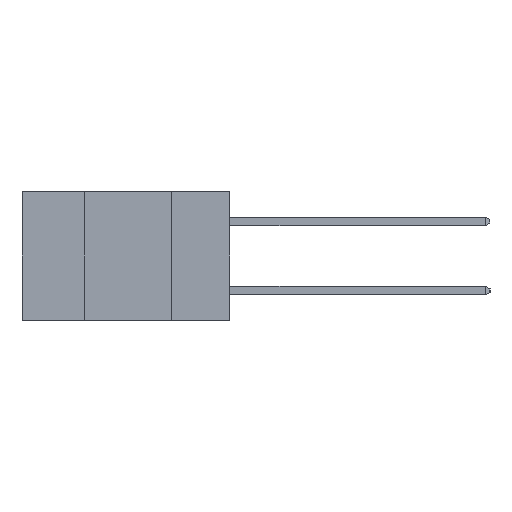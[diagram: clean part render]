
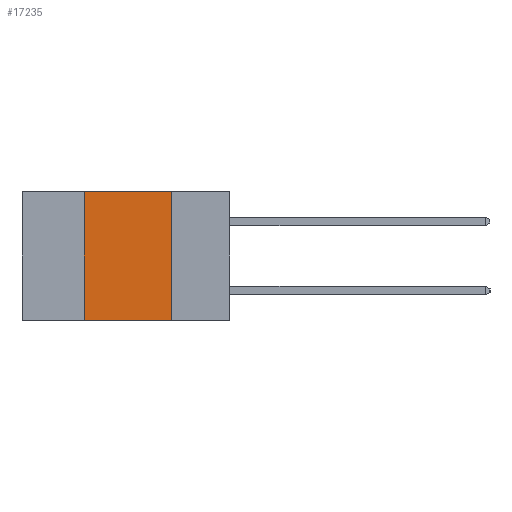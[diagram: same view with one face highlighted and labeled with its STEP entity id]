
A CAD part, left-side view. The second image highlights one B-rep face of the part: STEP entity #17235.
In plain terms, the highlighted planar face has unit normal (-1, 0, 0).
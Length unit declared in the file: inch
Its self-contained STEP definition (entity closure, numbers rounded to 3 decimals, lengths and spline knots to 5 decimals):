
#1787 = CARTESIAN_POINT ( 'NONE',  ( 0., 0.17, -0.37 ) ) ;
#2002 = LINE ( 'NONE', #13239, #11892 ) ;
#2721 = EDGE_CURVE ( 'NONE', #7994, #11828, #11859, .T. ) ;
#3943 = PLANE ( 'NONE',  #11125 ) ;
#5188 = VECTOR ( 'NONE', #9706, 39.37008 ) ;
#5270 = CARTESIAN_POINT ( 'NONE',  ( 0., 0.6, 0. ) ) ;
#5330 = DIRECTION ( 'NONE',  ( 0., 0., -1. ) ) ;
#7045 = ORIENTED_EDGE ( 'NONE', *, *, #13867, .F. ) ;
#7994 = VERTEX_POINT ( 'NONE', #9595 ) ;
#8025 = EDGE_CURVE ( 'NONE', #12094, #7994, #15851, .T. ) ;
#8326 = VECTOR ( 'NONE', #8555, 39.37008 ) ;
#8513 = CARTESIAN_POINT ( 'NONE',  ( 0., 0.6, 0. ) ) ;
#8555 = DIRECTION ( 'NONE',  ( 0., -1., 0. ) ) ;
#9113 = VERTEX_POINT ( 'NONE', #10528 ) ;
#9206 = LINE ( 'NONE', #1787, #12334 ) ;
#9595 = CARTESIAN_POINT ( 'NONE',  ( 0., 0.42, 0. ) ) ;
#9706 = DIRECTION ( 'NONE',  ( 0., 0., 1. ) ) ;
#9992 = CARTESIAN_POINT ( 'NONE',  ( 0., 0.17, 0. ) ) ;
#10528 = CARTESIAN_POINT ( 'NONE',  ( 0., 0.17, -0.37 ) ) ;
#10985 = CARTESIAN_POINT ( 'NONE',  ( 0., 0.42, -0.37 ) ) ;
#11112 = ORIENTED_EDGE ( 'NONE', *, *, #2721, .F. ) ;
#11125 = AXIS2_PLACEMENT_3D ( 'NONE', #5270, #13372, #5330 ) ;
#11564 = EDGE_LOOP ( 'NONE', ( #7045, #11112, #16531, #13802 ) ) ;
#11828 = VERTEX_POINT ( 'NONE', #9992 ) ;
#11859 = LINE ( 'NONE', #8513, #8326 ) ;
#11891 = DIRECTION ( 'NONE',  ( 0., -1., 0. ) ) ;
#11892 = VECTOR ( 'NONE', #11891, 39.37008 ) ;
#12094 = VERTEX_POINT ( 'NONE', #14474 ) ;
#12238 = FACE_OUTER_BOUND ( 'NONE', #11564, .T. ) ;
#12334 = VECTOR ( 'NONE', #16578, 39.37008 ) ;
#13239 = CARTESIAN_POINT ( 'NONE',  ( 0., 0.6, -0.37 ) ) ;
#13372 = DIRECTION ( 'NONE',  ( 1., 0., 0. ) ) ;
#13802 = ORIENTED_EDGE ( 'NONE', *, *, #14979, .T. ) ;
#13867 = EDGE_CURVE ( 'NONE', #11828, #9113, #9206, .T. ) ;
#14474 = CARTESIAN_POINT ( 'NONE',  ( 0., 0.42, -0.37 ) ) ;
#14979 = EDGE_CURVE ( 'NONE', #12094, #9113, #2002, .T. ) ;
#15851 = LINE ( 'NONE', #10985, #5188 ) ;
#16531 = ORIENTED_EDGE ( 'NONE', *, *, #8025, .F. ) ;
#16578 = DIRECTION ( 'NONE',  ( 0., 0., -1. ) ) ;
#17235 = ADVANCED_FACE ( 'NONE', ( #12238 ), #3943, .F. ) ;
